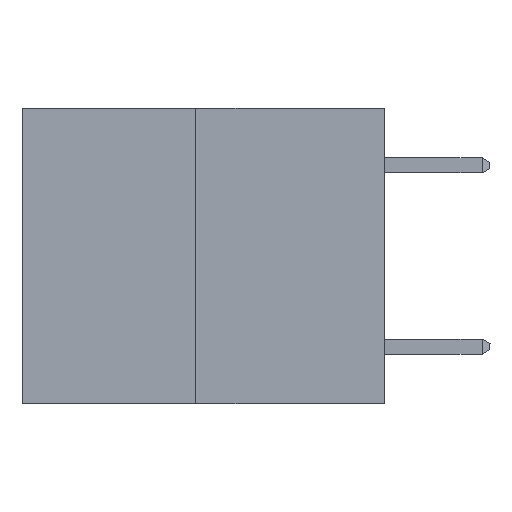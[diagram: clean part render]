
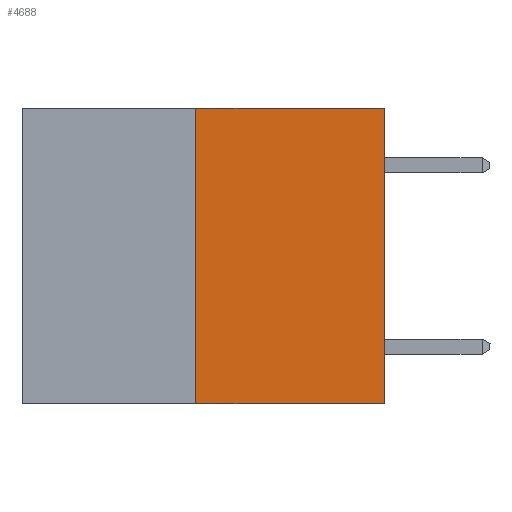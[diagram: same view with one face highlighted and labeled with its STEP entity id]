
A CAD part, left-side view. The second image highlights one B-rep face of the part: STEP entity #4688.
In plain terms, the highlighted planar face has unit normal (-1, 0, 0).
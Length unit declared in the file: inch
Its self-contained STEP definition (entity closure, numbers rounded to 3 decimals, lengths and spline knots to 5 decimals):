
#136 = VECTOR ( 'NONE', #2618, 39.37008 ) ;
#141 = CARTESIAN_POINT ( 'NONE',  ( 0., 0., -0.49 ) ) ;
#270 = VERTEX_POINT ( 'NONE', #5569 ) ;
#294 = DIRECTION ( 'NONE',  ( 0., -1., 0. ) ) ;
#1944 = CARTESIAN_POINT ( 'NONE',  ( 0., 0.6, -0.49 ) ) ;
#2273 = ORIENTED_EDGE ( 'NONE', *, *, #19678, .T. ) ;
#2434 = CARTESIAN_POINT ( 'NONE',  ( 0., 0.6, 0. ) ) ;
#2515 = DIRECTION ( 'NONE',  ( 1., 0., 0. ) ) ;
#2618 = DIRECTION ( 'NONE',  ( 0., -1., 0. ) ) ;
#3625 = VERTEX_POINT ( 'NONE', #16138 ) ;
#4688 = ADVANCED_FACE ( 'NONE', ( #11335 ), #7685, .F. ) ;
#4742 = ORIENTED_EDGE ( 'NONE', *, *, #19660, .F. ) ;
#5569 = CARTESIAN_POINT ( 'NONE',  ( 0., 0., 0. ) ) ;
#7685 = PLANE ( 'NONE',  #19041 ) ;
#7757 = EDGE_CURVE ( 'NONE', #9550, #13686, #9976, .T. ) ;
#7892 = ORIENTED_EDGE ( 'NONE', *, *, #7757, .T. ) ;
#8123 = LINE ( 'NONE', #16306, #136 ) ;
#9074 = ORIENTED_EDGE ( 'NONE', *, *, #9701, .F. ) ;
#9494 = CARTESIAN_POINT ( 'NONE',  ( 0., 0., 0. ) ) ;
#9550 = VERTEX_POINT ( 'NONE', #14297 ) ;
#9701 = EDGE_CURVE ( 'NONE', #9550, #3625, #13375, .T. ) ;
#9976 = LINE ( 'NONE', #1944, #21267 ) ;
#11335 = FACE_OUTER_BOUND ( 'NONE', #16928, .T. ) ;
#11797 = VECTOR ( 'NONE', #12402, 39.37008 ) ;
#12402 = DIRECTION ( 'NONE',  ( 0., 0., 1. ) ) ;
#12655 = DIRECTION ( 'NONE',  ( 0., 0., 1. ) ) ;
#13375 = LINE ( 'NONE', #15742, #11797 ) ;
#13686 = VERTEX_POINT ( 'NONE', #141 ) ;
#14297 = CARTESIAN_POINT ( 'NONE',  ( 0., 0.312, -0.49 ) ) ;
#14506 = LINE ( 'NONE', #9494, #18287 ) ;
#15742 = CARTESIAN_POINT ( 'NONE',  ( 0., 0.312, -0.49 ) ) ;
#16138 = CARTESIAN_POINT ( 'NONE',  ( 0., 0.312, 0. ) ) ;
#16306 = CARTESIAN_POINT ( 'NONE',  ( 0., 0.6, 0. ) ) ;
#16928 = EDGE_LOOP ( 'NONE', ( #9074, #7892, #2273, #4742 ) ) ;
#17860 = DIRECTION ( 'NONE',  ( 0., 0., -1. ) ) ;
#18287 = VECTOR ( 'NONE', #12655, 39.37008 ) ;
#19041 = AXIS2_PLACEMENT_3D ( 'NONE', #2434, #2515, #17860 ) ;
#19660 = EDGE_CURVE ( 'NONE', #3625, #270, #8123, .T. ) ;
#19678 = EDGE_CURVE ( 'NONE', #13686, #270, #14506, .T. ) ;
#21267 = VECTOR ( 'NONE', #294, 39.37008 ) ;
